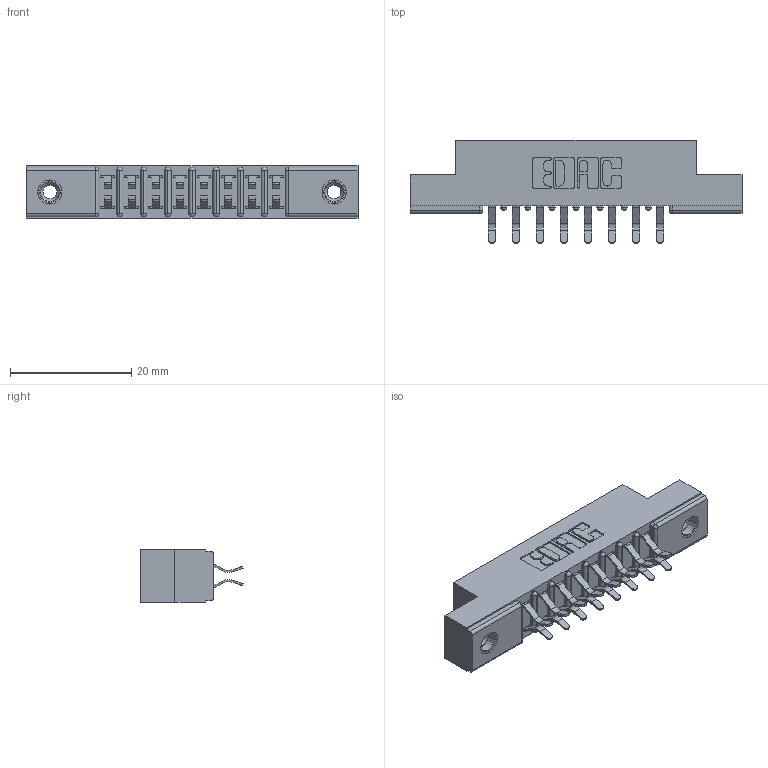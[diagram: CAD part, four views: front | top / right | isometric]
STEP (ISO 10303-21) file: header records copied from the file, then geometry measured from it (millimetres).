
FILE_DESCRIPTION (( 'STEP AP203' ), '1' );
FILE_NAME ('307-016-556-208.STEP', '2019-09-05T19:28:49', ( '' ), ( '' ), 'SwSTEP 2.0', 'SolidWorks 2016', '' );
FILE_SCHEMA (( 'CONFIG_CONTROL_DESIGN' ));
Length unit declared in the file: inch
Products named in the file (4): 307 Part_.156 Dia Mounting Holes; 307-016-556-208; 345-250-001_345-250-003-102; 307-290-001_556
Assembly tree (19 placements, depth 2):
  307-016-556-208
    307 Part_.156 Dia Mounting Holes
    307-290-001_556  x16
    345-250-001_345-250-003-102  x2
Bounding box: 54.71 x 16.97 x 8.71 mm (x, y, z)
Volume: 3570.9 mm3; surface area: 5582.6 mm2
Topology: 19 solids, 19 shells, 987 faces, 2731 edges, 1766 vertices
Faces by surface type: plane 630, cylinder 323, sphere 18, cone 12, torus 4
Entity records: 12595 total; most frequent: CARTESIAN_POINT 2055, DIRECTION 2037, ORIENTED_EDGE 2026, EDGE_CURVE 1013, LINE 761, VECTOR 761, VERTEX_POINT 656, AXIS2_PLACEMENT_3D 638
